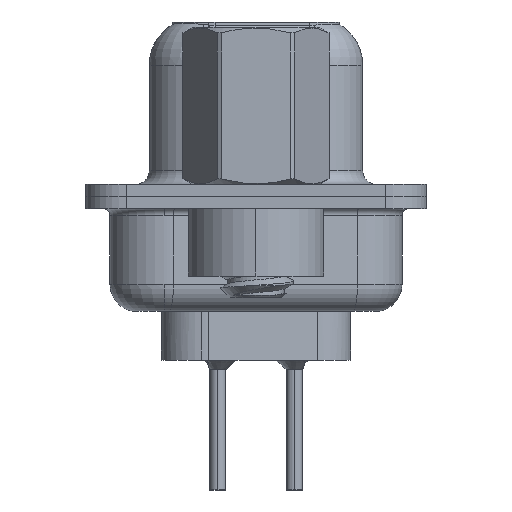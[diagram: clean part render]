
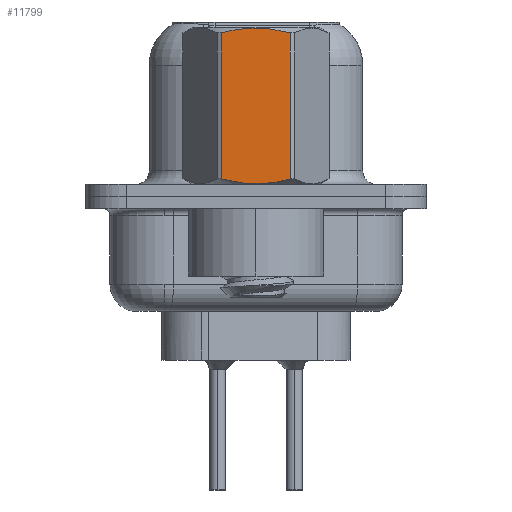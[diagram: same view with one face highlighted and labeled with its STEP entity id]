
A CAD part, left-side view. The second image highlights one B-rep face of the part: STEP entity #11799.
In plain terms, the highlighted planar face has unit normal (-1, 0, 0).
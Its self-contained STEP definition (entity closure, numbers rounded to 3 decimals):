
#484 = VERTEX_POINT ( 'NONE', #7603 ) ;
#1700 = DIRECTION ( 'NONE',  ( -1., 0., 0. ) ) ;
#1710 = EDGE_CURVE ( 'NONE', #26920, #484, #4839, .T. ) ;
#2000 = FACE_OUTER_BOUND ( 'NONE', #14876, .T. ) ;
#2097 = CARTESIAN_POINT ( 'NONE',  ( -2.381, 0.215, 0.468 ) ) ;
#2697 = CARTESIAN_POINT ( 'NONE',  ( -2.381, 1.273, 3.792 ) ) ;
#2954 = LINE ( 'NONE', #16360, #24007 ) ;
#2960 = EDGE_CURVE ( 'NONE', #24739, #26920, #2954, .T. ) ;
#4127 = VERTEX_POINT ( 'NONE', #7351 ) ;
#4839 = B_SPLINE_CURVE_WITH_KNOTS ( 'NONE', 3,
 ( #12160, #10002, #11723, #7375, #9708, #22806, #20609, #22951, #20467, #7085 ),
 .UNSPECIFIED., .F., .F.,
 ( 4, 2, 2, 2, 4 ),
 ( 0.001, 0.002, 0.002, 0.003, 0.004 ),
 .UNSPECIFIED. ) ;
#4886 = LINE ( 'NONE', #2697, #26127 ) ;
#7085 = CARTESIAN_POINT ( 'NONE',  ( -2.381, 1.273, 6.048 ) ) ;
#7351 = CARTESIAN_POINT ( 'NONE',  ( -2.381, 1.273, 0.652 ) ) ;
#7375 = CARTESIAN_POINT ( 'NONE',  ( -2.381, -0.432, 6.215 ) ) ;
#7603 = CARTESIAN_POINT ( 'NONE',  ( -2.381, 1.273, 6.048 ) ) ;
#8558 = CARTESIAN_POINT ( 'NONE',  ( -2.381, 1.065, 0.596 ) ) ;
#9679 = DIRECTION ( 'NONE',  ( 0., 0., 1. ) ) ;
#9708 = CARTESIAN_POINT ( 'NONE',  ( -2.381, -0.215, 6.232 ) ) ;
#10002 = CARTESIAN_POINT ( 'NONE',  ( -2.381, -1.066, 6.104 ) ) ;
#10291 = CARTESIAN_POINT ( 'NONE',  ( -2.381, 1.273, 0.652 ) ) ;
#10627 = DIRECTION ( 'NONE',  ( 0., -1., 0. ) ) ;
#11723 = CARTESIAN_POINT ( 'NONE',  ( -2.381, -0.858, 6.15 ) ) ;
#11799 = ADVANCED_FACE ( 'NONE', ( #2000 ), #17311, .T. ) ;
#12160 = CARTESIAN_POINT ( 'NONE',  ( -2.381, -1.273, 6.048 ) ) ;
#12383 = B_SPLINE_CURVE_WITH_KNOTS ( 'NONE', 3,
 ( #10291, #8558, #21652, #19598, #2097, #28780, #15230, #23986, #24405, #17699 ),
 .UNSPECIFIED., .F., .F.,
 ( 4, 2, 2, 2, 4 ),
 ( 0.003, 0.003, 0.004, 0.004, 0.005 ),
 .UNSPECIFIED. ) ;
#13490 = DIRECTION ( 'NONE',  ( 0., 0., -1. ) ) ;
#13883 = CARTESIAN_POINT ( 'NONE',  ( -2.381, -1.273, 0.652 ) ) ;
#14275 = ORIENTED_EDGE ( 'NONE', *, *, #1710, .T. ) ;
#14876 = EDGE_LOOP ( 'NONE', ( #25715, #17507, #14275, #16044 ) ) ;
#15230 = CARTESIAN_POINT ( 'NONE',  ( -2.381, -0.432, 0.485 ) ) ;
#16044 = ORIENTED_EDGE ( 'NONE', *, *, #21688, .T. ) ;
#16360 = CARTESIAN_POINT ( 'NONE',  ( -2.381, -1.273, 3.792 ) ) ;
#17311 = PLANE ( 'NONE',  #19543 ) ;
#17507 = ORIENTED_EDGE ( 'NONE', *, *, #2960, .T. ) ;
#17699 = CARTESIAN_POINT ( 'NONE',  ( -2.381, -1.273, 0.652 ) ) ;
#19543 = AXIS2_PLACEMENT_3D ( 'NONE', #21700, #1700, #10627 ) ;
#19598 = CARTESIAN_POINT ( 'NONE',  ( -2.381, 0.428, 0.485 ) ) ;
#20113 = CARTESIAN_POINT ( 'NONE',  ( -2.381, -1.273, 6.048 ) ) ;
#20467 = CARTESIAN_POINT ( 'NONE',  ( -2.381, 1.065, 6.104 ) ) ;
#20609 = CARTESIAN_POINT ( 'NONE',  ( -2.381, 0.428, 6.215 ) ) ;
#21652 = CARTESIAN_POINT ( 'NONE',  ( -2.381, 0.853, 0.549 ) ) ;
#21688 = EDGE_CURVE ( 'NONE', #484, #4127, #4886, .T. ) ;
#21700 = CARTESIAN_POINT ( 'NONE',  ( -2.381, 1.375, -3.75 ) ) ;
#22806 = CARTESIAN_POINT ( 'NONE',  ( -2.381, 0.215, 6.232 ) ) ;
#22951 = CARTESIAN_POINT ( 'NONE',  ( -2.381, 0.853, 6.151 ) ) ;
#23986 = CARTESIAN_POINT ( 'NONE',  ( -2.381, -0.858, 0.55 ) ) ;
#24007 = VECTOR ( 'NONE', #9679, 1000. ) ;
#24405 = CARTESIAN_POINT ( 'NONE',  ( -2.381, -1.066, 0.596 ) ) ;
#24561 = EDGE_CURVE ( 'NONE', #4127, #24739, #12383, .T. ) ;
#24739 = VERTEX_POINT ( 'NONE', #13883 ) ;
#25715 = ORIENTED_EDGE ( 'NONE', *, *, #24561, .T. ) ;
#26127 = VECTOR ( 'NONE', #13490, 1000. ) ;
#26920 = VERTEX_POINT ( 'NONE', #20113 ) ;
#28780 = CARTESIAN_POINT ( 'NONE',  ( -2.381, -0.215, 0.468 ) ) ;
